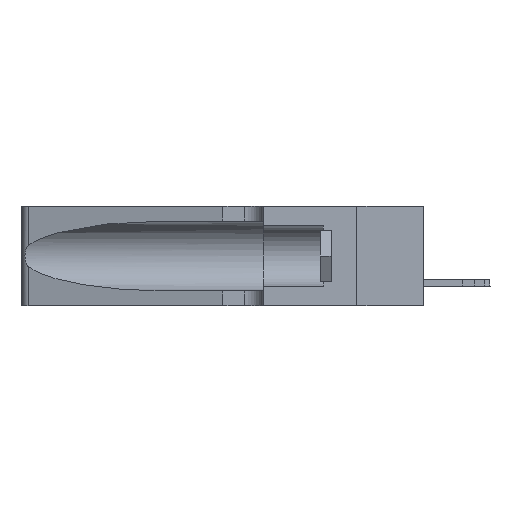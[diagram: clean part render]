
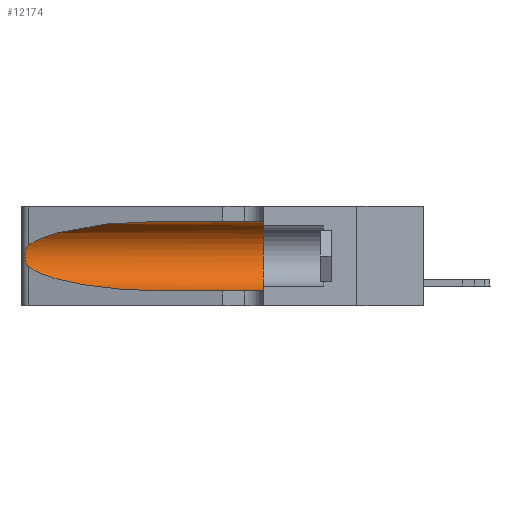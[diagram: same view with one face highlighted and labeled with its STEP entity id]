
A CAD part, left-side view. The second image highlights one B-rep face of the part: STEP entity #12174.
In plain terms, the highlighted cylindrical face has radius 3.308 mm (diameter 6.617 mm), a partial arc.
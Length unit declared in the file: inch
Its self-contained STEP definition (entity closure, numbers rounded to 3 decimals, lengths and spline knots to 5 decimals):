
#170 = EDGE_CURVE ( 'NONE', #14387, #15865, #19036, .T. ) ;
#182 = DIRECTION ( 'NONE',  ( 0., -1., 0. ) ) ;
#230 = CARTESIAN_POINT ( 'NONE',  ( 0.25487, 1.22718, 0.22369 ) ) ;
#427 = CARTESIAN_POINT ( 'NONE',  ( 0.1305, 1.61858, 0.05475 ) ) ;
#556 = AXIS2_PLACEMENT_3D ( 'NONE', #12766, #182, #5777 ) ;
#1256 = ORIENTED_EDGE ( 'NONE', *, *, #7097, .F. ) ;
#1667 = CARTESIAN_POINT ( 'NONE',  ( 0.25487, 1.22718, 0.22369 ) ) ;
#2206 = VECTOR ( 'NONE', #11393, 39.37008 ) ;
#2426 = ORIENTED_EDGE ( 'NONE', *, *, #13208, .F. ) ;
#3211 = EDGE_CURVE ( 'NONE', #19315, #17439, #4567, .T. ) ;
#4476 = LINE ( 'NONE', #427, #7791 ) ;
#4567 =( BOUNDED_CURVE ( )  B_SPLINE_CURVE ( 3, ( #10531, #7116, #8678, #10672 ),
 .UNSPECIFIED., .F., .F. ) 
 B_SPLINE_CURVE_WITH_KNOTS ( ( 4, 4 ),
 ( 3.44316, 4.71239 ),
 .UNSPECIFIED. ) 
 CURVE ( )  GEOMETRIC_REPRESENTATION_ITEM ( )  RATIONAL_B_SPLINE_CURVE ( ( 1., 0.87, 0.87, 1. ) ) 
 REPRESENTATION_ITEM ( '' )  );
#4968 = B_SPLINE_CURVE_WITH_KNOTS ( 'NONE', 3,
 ( #1667, #12184, #15789, #14143, #21382, #16015, #5357, #17834, #7271, #10908, #10841, #12797, #5658, #11063 ),
 .UNSPECIFIED., .F., .F.,
 ( 4, 2, 2, 2, 2, 2, 4 ),
 ( 0., 0.00027, 0.00053, 0.00107, 0.0016, 0.00187, 0.00214 ),
 .UNSPECIFIED. ) ;
#5357 = CARTESIAN_POINT ( 'NONE',  ( 0.26075, 1.23896, 0.19203 ) ) ;
#5658 = CARTESIAN_POINT ( 'NONE',  ( 0.25555, 1.22993, 0.14849 ) ) ;
#5777 = DIRECTION ( 'NONE',  ( 0., 0., -1. ) ) ;
#6002 = CARTESIAN_POINT ( 'NONE',  ( 0.25487, 1.22718, 0.14631 ) ) ;
#6160 = LINE ( 'NONE', #20274, #2206 ) ;
#7097 = EDGE_CURVE ( 'NONE', #14387, #19696, #6160, .T. ) ;
#7116 = CARTESIAN_POINT ( 'NONE',  ( 0.2373, 1.15595, 0.08982 ) ) ;
#7269 = CARTESIAN_POINT ( 'NONE',  ( 0.1305, 0.72297, 0.31525 ) ) ;
#7271 = CARTESIAN_POINT ( 'NONE',  ( 0.26017, 1.23833, 0.17102 ) ) ;
#7519 = CARTESIAN_POINT ( 'NONE',  ( 0.1305, 0.35, 0.05475 ) ) ;
#7618 = CARTESIAN_POINT ( 'NONE',  ( 0.1305, 0.35, 0.31525 ) ) ;
#7791 = VECTOR ( 'NONE', #12938, 39.37008 ) ;
#8547 = EDGE_LOOP ( 'NONE', ( #17962, #19818, #21407, #10941, #2426, #1256 ) ) ;
#8593 = CYLINDRICAL_SURFACE ( 'NONE', #556, 0.13025 ) ;
#8678 = CARTESIAN_POINT ( 'NONE',  ( 0.18966, 0.96281, 0.05475 ) ) ;
#10531 = CARTESIAN_POINT ( 'NONE',  ( 0.25487, 1.22718, 0.14631 ) ) ;
#10589 = EDGE_CURVE ( 'NONE', #17439, #12792, #4476, .T. ) ;
#10609 = CARTESIAN_POINT ( 'NONE',  ( 0.1305, 0.35, 0.185 ) ) ;
#10672 = CARTESIAN_POINT ( 'NONE',  ( 0.1305, 0.72297, 0.05475 ) ) ;
#10841 = CARTESIAN_POINT ( 'NONE',  ( 0.25789, 1.23486, 0.15765 ) ) ;
#10859 = CARTESIAN_POINT ( 'NONE',  ( 0.18966, 0.96281, 0.31525 ) ) ;
#10908 = CARTESIAN_POINT ( 'NONE',  ( 0.25856, 1.23593, 0.16098 ) ) ;
#10930 = CARTESIAN_POINT ( 'NONE',  ( 0.1305, 0.72297, 0.31525 ) ) ;
#10941 = ORIENTED_EDGE ( 'NONE', *, *, #10589, .T. ) ;
#11063 = CARTESIAN_POINT ( 'NONE',  ( 0.25487, 1.22718, 0.14631 ) ) ;
#11393 = DIRECTION ( 'NONE',  ( 0., -1., 0. ) ) ;
#12174 = ADVANCED_FACE ( 'NONE', ( #21488 ), #8593, .F. ) ;
#12184 = CARTESIAN_POINT ( 'NONE',  ( 0.25555, 1.22994, 0.2215 ) ) ;
#12766 = CARTESIAN_POINT ( 'NONE',  ( 0.1305, 1.61858, 0.185 ) ) ;
#12792 = VERTEX_POINT ( 'NONE', #7519 ) ;
#12797 = CARTESIAN_POINT ( 'NONE',  ( 0.25639, 1.23186, 0.15144 ) ) ;
#12938 = DIRECTION ( 'NONE',  ( 0., -1., 0. ) ) ;
#13208 = EDGE_CURVE ( 'NONE', #19696, #12792, #22815, .T. ) ;
#14143 = CARTESIAN_POINT ( 'NONE',  ( 0.25787, 1.23484, 0.2124 ) ) ;
#14387 = VERTEX_POINT ( 'NONE', #7269 ) ;
#15789 = CARTESIAN_POINT ( 'NONE',  ( 0.25639, 1.23184, 0.21858 ) ) ;
#15865 = VERTEX_POINT ( 'NONE', #20796 ) ;
#16015 = CARTESIAN_POINT ( 'NONE',  ( 0.26018, 1.23835, 0.19895 ) ) ;
#16910 = AXIS2_PLACEMENT_3D ( 'NONE', #10609, #21308, #21452 ) ;
#17439 = VERTEX_POINT ( 'NONE', #22094 ) ;
#17834 = CARTESIAN_POINT ( 'NONE',  ( 0.26075, 1.23896, 0.178 ) ) ;
#17962 = ORIENTED_EDGE ( 'NONE', *, *, #170, .T. ) ;
#19036 =( BOUNDED_CURVE ( )  B_SPLINE_CURVE ( 3, ( #10930, #10859, #20141, #230 ),
 .UNSPECIFIED., .F., .T. ) 
 B_SPLINE_CURVE_WITH_KNOTS ( ( 4, 4 ),
 ( 1.5708, 2.84003 ),
 .UNSPECIFIED. ) 
 CURVE ( )  GEOMETRIC_REPRESENTATION_ITEM ( )  RATIONAL_B_SPLINE_CURVE ( ( 1., 0.87, 0.87, 1. ) ) 
 REPRESENTATION_ITEM ( '' )  );
#19315 = VERTEX_POINT ( 'NONE', #6002 ) ;
#19696 = VERTEX_POINT ( 'NONE', #7618 ) ;
#19818 = ORIENTED_EDGE ( 'NONE', *, *, #21661, .T. ) ;
#20141 = CARTESIAN_POINT ( 'NONE',  ( 0.2373, 1.15595, 0.28018 ) ) ;
#20274 = CARTESIAN_POINT ( 'NONE',  ( 0.1305, 1.61858, 0.31525 ) ) ;
#20796 = CARTESIAN_POINT ( 'NONE',  ( 0.25487, 1.22718, 0.22369 ) ) ;
#21308 = DIRECTION ( 'NONE',  ( 0., 1., 0. ) ) ;
#21382 = CARTESIAN_POINT ( 'NONE',  ( 0.25854, 1.2359, 0.20912 ) ) ;
#21407 = ORIENTED_EDGE ( 'NONE', *, *, #3211, .T. ) ;
#21452 = DIRECTION ( 'NONE',  ( 0., 0., 1. ) ) ;
#21488 = FACE_OUTER_BOUND ( 'NONE', #8547, .T. ) ;
#21661 = EDGE_CURVE ( 'NONE', #15865, #19315, #4968, .T. ) ;
#22094 = CARTESIAN_POINT ( 'NONE',  ( 0.1305, 0.72297, 0.05475 ) ) ;
#22815 = CIRCLE ( 'NONE', #16910, 0.13025 ) ;
